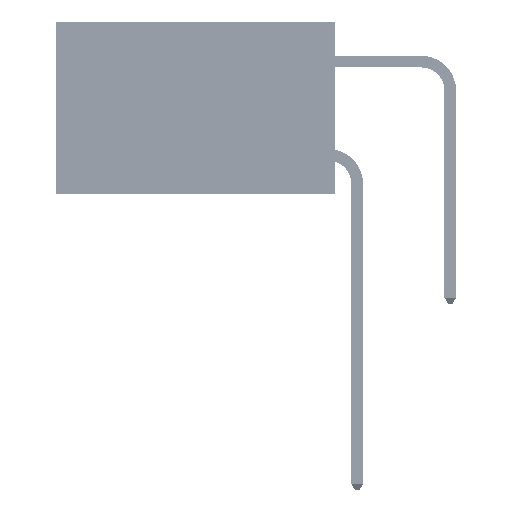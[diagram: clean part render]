
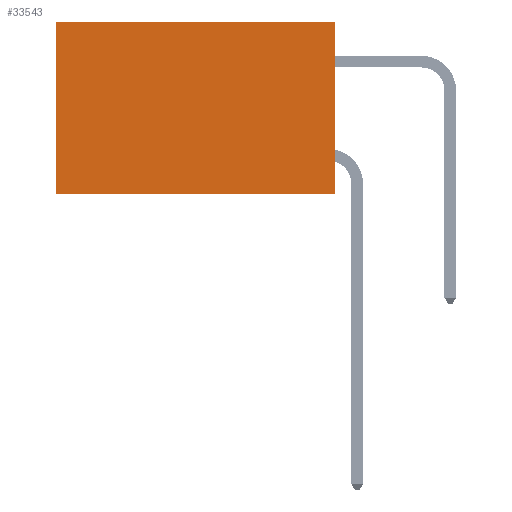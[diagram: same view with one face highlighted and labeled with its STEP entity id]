
A CAD part, left-side view. The second image highlights one B-rep face of the part: STEP entity #33543.
In plain terms, the highlighted planar face has unit normal (-1, 0, 0).
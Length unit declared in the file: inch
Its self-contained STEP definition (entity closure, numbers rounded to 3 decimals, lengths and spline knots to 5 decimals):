
#1039 = VERTEX_POINT ( 'NONE', #10616 ) ;
#1219 = DIRECTION ( 'NONE',  ( 0., 1., 0. ) ) ;
#1479 = LINE ( 'NONE', #14330, #11031 ) ;
#3365 = PLANE ( 'NONE',  #14676 ) ;
#8084 = CARTESIAN_POINT ( 'NONE',  ( 0.2875, 0., 0. ) ) ;
#8397 = EDGE_CURVE ( 'NONE', #20723, #39421, #36198, .T. ) ;
#10275 = EDGE_CURVE ( 'NONE', #20723, #27254, #31536, .T. ) ;
#10577 = DIRECTION ( 'NONE',  ( 0., 0., -1. ) ) ;
#10616 = CARTESIAN_POINT ( 'NONE',  ( 0.2875, 0.6, -0.37 ) ) ;
#11031 = VECTOR ( 'NONE', #35530, 39.37008 ) ;
#12566 = VECTOR ( 'NONE', #1219, 39.37008 ) ;
#12748 = VECTOR ( 'NONE', #36423, 39.37008 ) ;
#13390 = EDGE_CURVE ( 'NONE', #39421, #1039, #1479, .T. ) ;
#13625 = ORIENTED_EDGE ( 'NONE', *, *, #46054, .F. ) ;
#14330 = CARTESIAN_POINT ( 'NONE',  ( 0.2875, 0.6, 0. ) ) ;
#14676 = AXIS2_PLACEMENT_3D ( 'NONE', #28254, #31745, #10577 ) ;
#19767 = CARTESIAN_POINT ( 'NONE',  ( 0.2875, 0., 0. ) ) ;
#19909 = FACE_OUTER_BOUND ( 'NONE', #39041, .T. ) ;
#20723 = VERTEX_POINT ( 'NONE', #33940 ) ;
#26147 = CARTESIAN_POINT ( 'NONE',  ( 0.2875, 0., -0.37 ) ) ;
#26795 = VECTOR ( 'NONE', #37586, 39.37008 ) ;
#27112 = ORIENTED_EDGE ( 'NONE', *, *, #8397, .T. ) ;
#27254 = VERTEX_POINT ( 'NONE', #32968 ) ;
#28254 = CARTESIAN_POINT ( 'NONE',  ( 0.2875, 0., 0. ) ) ;
#29698 = CARTESIAN_POINT ( 'NONE',  ( 0.2875, 0.6, 0. ) ) ;
#31536 = LINE ( 'NONE', #8084, #12748 ) ;
#31745 = DIRECTION ( 'NONE',  ( 1., 0., 0. ) ) ;
#32163 = ORIENTED_EDGE ( 'NONE', *, *, #10275, .F. ) ;
#32968 = CARTESIAN_POINT ( 'NONE',  ( 0.2875, 0., -0.37 ) ) ;
#33543 = ADVANCED_FACE ( 'NONE', ( #19909 ), #3365, .F. ) ;
#33940 = CARTESIAN_POINT ( 'NONE',  ( 0.2875, 0., 0. ) ) ;
#35530 = DIRECTION ( 'NONE',  ( 0., 0., -1. ) ) ;
#36198 = LINE ( 'NONE', #19767, #26795 ) ;
#36423 = DIRECTION ( 'NONE',  ( 0., 0., -1. ) ) ;
#37586 = DIRECTION ( 'NONE',  ( 0., 1., 0. ) ) ;
#37806 = ORIENTED_EDGE ( 'NONE', *, *, #13390, .T. ) ;
#38595 = LINE ( 'NONE', #26147, #12566 ) ;
#39041 = EDGE_LOOP ( 'NONE', ( #37806, #13625, #32163, #27112 ) ) ;
#39421 = VERTEX_POINT ( 'NONE', #29698 ) ;
#46054 = EDGE_CURVE ( 'NONE', #27254, #1039, #38595, .T. ) ;
